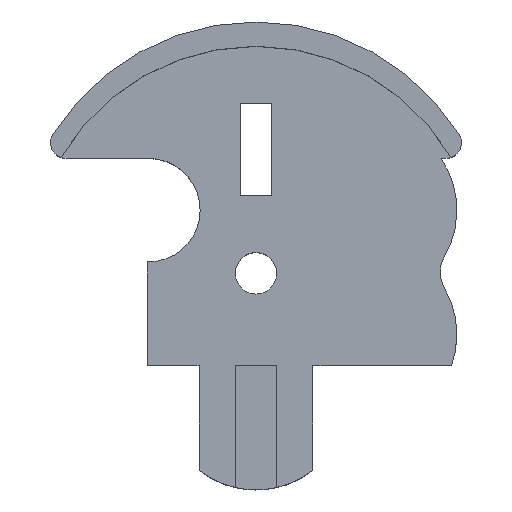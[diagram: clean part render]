
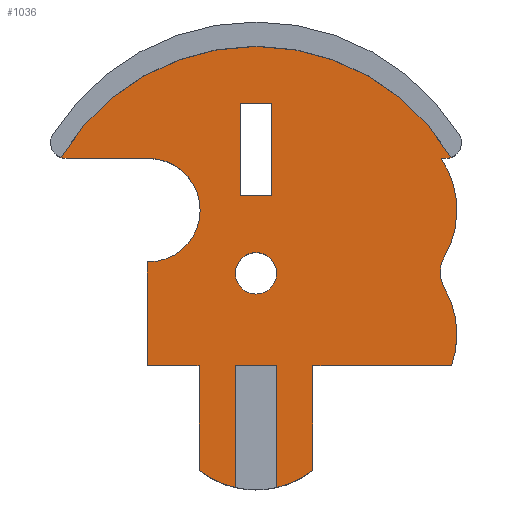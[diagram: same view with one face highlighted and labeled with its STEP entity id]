
A CAD part, top view. The second image highlights one B-rep face of the part: STEP entity #1036.
In plain terms, the highlighted planar face has unit normal (0, 0, 1).
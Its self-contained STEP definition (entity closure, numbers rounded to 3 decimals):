
#73=CARTESIAN_POINT('',(18.831,-0.817,10.0));
#74=VERTEX_POINT('',#73);
#75=CARTESIAN_POINT('',(-18.831,-0.817,10.0));
#76=VERTEX_POINT('',#75);
#77=CARTESIAN_POINT('',(0.0,-11.997,10.0));
#78=DIRECTION('',(0.0,0.0,1.0));
#79=DIRECTION('',(-0.86,-0.51,0.0));
#80=AXIS2_PLACEMENT_3D('',#77,#78,#79);
#81=CIRCLE('',#80,21.9);
#82=EDGE_CURVE('',#74,#76,#81,.T.);
#205=CARTESIAN_POINT('',(-1.998,-32.676,10.0));
#206=VERTEX_POINT('',#205);
#207=CARTESIAN_POINT('',(-1.998,-20.9,10.0));
#208=VERTEX_POINT('',#207);
#209=CARTESIAN_POINT('',(-1.998,-32.676,10.0));
#210=DIRECTION('',(0.0,1.0,0.0));
#211=VECTOR('',#210,11.775);
#212=LINE('',#209,#211);
#213=EDGE_CURVE('',#206,#208,#212,.T.);
#248=CARTESIAN_POINT('',(2.002,-20.9,10.0));
#249=VERTEX_POINT('',#248);
#250=CARTESIAN_POINT('',(2.002,-32.675,10.0));
#251=VERTEX_POINT('',#250);
#252=CARTESIAN_POINT('',(2.002,-20.9,10.0));
#253=DIRECTION('',(0.0,-1.0,0.0));
#254=VECTOR('',#253,11.774);
#255=LINE('',#252,#254);
#256=EDGE_CURVE('',#249,#251,#255,.T.);
#291=CARTESIAN_POINT('',(-1.998,-20.9,10.0));
#292=DIRECTION('',(1.0,0.0,0.0));
#293=VECTOR('',#292,4.0);
#294=LINE('',#291,#293);
#295=EDGE_CURVE('',#208,#249,#294,.T.);
#334=CARTESIAN_POINT('',(-5.5,-31.024,10.0));
#335=VERTEX_POINT('',#334);
#336=CARTESIAN_POINT('',(0.,-23.9,10.0));
#337=DIRECTION('',(0.0,0.0,1.0));
#338=DIRECTION('',(-0.611,-0.792,0.0));
#339=AXIS2_PLACEMENT_3D('',#336,#337,#338);
#340=CIRCLE('',#339,9.);
#341=EDGE_CURVE('',#335,#206,#340,.T.);
#360=CARTESIAN_POINT('',(5.5,-31.024,10.0));
#361=VERTEX_POINT('',#360);
#368=CARTESIAN_POINT('',(0.,-23.9,10.0));
#369=DIRECTION('',(0.0,0.0,1.0));
#370=DIRECTION('',(-0.611,-0.792,0.0));
#371=AXIS2_PLACEMENT_3D('',#368,#369,#370);
#372=CIRCLE('',#371,9.);
#373=EDGE_CURVE('',#251,#361,#372,.T.);
#393=CARTESIAN_POINT('',(1.5,4.426,10.0));
#394=VERTEX_POINT('',#393);
#401=CARTESIAN_POINT('',(-1.5,4.426,10.0));
#402=VERTEX_POINT('',#401);
#403=CARTESIAN_POINT('',(-1.5,4.426,10.0));
#404=DIRECTION('',(1.0,0.0,0.0));
#405=VECTOR('',#404,3.);
#406=LINE('',#403,#405);
#407=EDGE_CURVE('',#402,#394,#406,.T.);
#431=CARTESIAN_POINT('',(1.5,-4.532,10.0));
#432=VERTEX_POINT('',#431);
#439=CARTESIAN_POINT('',(1.5,4.426,10.0));
#440=DIRECTION('',(0.0,-1.0,0.0));
#441=VECTOR('',#440,8.958);
#442=LINE('',#439,#441);
#443=EDGE_CURVE('',#394,#432,#442,.T.);
#462=CARTESIAN_POINT('',(-1.5,-4.532,10.0));
#463=VERTEX_POINT('',#462);
#470=CARTESIAN_POINT('',(1.5,-4.532,10.0));
#471=DIRECTION('',(-1.0,0.0,0.0));
#472=VECTOR('',#471,3.);
#473=LINE('',#470,#472);
#474=EDGE_CURVE('',#432,#463,#473,.T.);
#492=CARTESIAN_POINT('',(-1.5,-4.532,10.0));
#493=DIRECTION('',(0.0,1.0,0.0));
#494=VECTOR('',#493,8.958);
#495=LINE('',#492,#494);
#496=EDGE_CURVE('',#463,#402,#495,.T.);
#507=CARTESIAN_POINT('',(2.0,-11.997,10.0));
#508=VERTEX_POINT('',#507);
#509=CARTESIAN_POINT('',(0.0,-11.997,10.0));
#510=DIRECTION('',(0.0,0.0,-1.0));
#511=DIRECTION('',(-1.0,0.0,0.0));
#512=AXIS2_PLACEMENT_3D('',#509,#510,#511);
#513=CIRCLE('',#512,2.0);
#514=EDGE_CURVE('',#508,#508,#513,.T.);
#545=CARTESIAN_POINT('',(18.878,-20.9,10.0));
#546=VERTEX_POINT('',#545);
#553=CARTESIAN_POINT('',(5.5,-20.9,10.0));
#554=VERTEX_POINT('',#553);
#555=CARTESIAN_POINT('',(5.5,-20.9,10.0));
#556=DIRECTION('',(1.0,0.0,0.0));
#557=VECTOR('',#556,13.378);
#558=LINE('',#555,#557);
#559=EDGE_CURVE('',#554,#546,#558,.T.);
#582=CARTESIAN_POINT('',(5.5,-31.024,10.0));
#583=DIRECTION('',(0.0,1.0,0.0));
#584=VECTOR('',#583,10.124);
#585=LINE('',#582,#584);
#586=EDGE_CURVE('',#361,#554,#585,.T.);
#609=CARTESIAN_POINT('',(-5.5,-20.9,10.0));
#610=VERTEX_POINT('',#609);
#611=CARTESIAN_POINT('',(-5.5,-20.9,10.0));
#612=DIRECTION('',(0.0,-1.0,0.0));
#613=VECTOR('',#612,10.124);
#614=LINE('',#611,#613);
#615=EDGE_CURVE('',#610,#335,#614,.T.);
#643=CARTESIAN_POINT('',(-10.5,-20.9,10.0));
#644=VERTEX_POINT('',#643);
#645=CARTESIAN_POINT('',(-10.5,-20.9,10.0));
#646=DIRECTION('',(1.0,0.0,0.0));
#647=VECTOR('',#646,5.);
#648=LINE('',#645,#647);
#649=EDGE_CURVE('',#644,#610,#648,.T.);
#674=CARTESIAN_POINT('',(-10.5,-10.9,10.0));
#675=VERTEX_POINT('',#674);
#676=CARTESIAN_POINT('',(-10.5,-10.9,10.0));
#677=DIRECTION('',(0.0,-1.0,0.0));
#678=VECTOR('',#677,10.);
#679=LINE('',#676,#678);
#680=EDGE_CURVE('',#675,#644,#679,.T.);
#705=CARTESIAN_POINT('',(-10.392,-10.9,10.0));
#706=VERTEX_POINT('',#705);
#707=CARTESIAN_POINT('',(-10.392,-10.9,10.0));
#708=DIRECTION('',(-1.0,0.0,0.0));
#709=VECTOR('',#708,0.108);
#710=LINE('',#707,#709);
#711=EDGE_CURVE('',#706,#675,#710,.T.);
#737=CARTESIAN_POINT('',(-10.392,-0.9,10.0));
#738=VERTEX_POINT('',#737);
#739=CARTESIAN_POINT('',(-10.392,-5.9,10.0));
#740=DIRECTION('',(0.0,0.0,-1.0));
#741=DIRECTION('',(0.0,1.0,0.0));
#742=AXIS2_PLACEMENT_3D('',#739,#740,#741);
#743=CIRCLE('',#742,5.);
#744=EDGE_CURVE('',#738,#706,#743,.T.);
#769=CARTESIAN_POINT('',(-18.34,-0.9,10.0));
#770=VERTEX_POINT('',#769);
#771=CARTESIAN_POINT('',(-18.34,-0.9,10.0));
#772=DIRECTION('',(1.0,0.0,0.0));
#773=VECTOR('',#772,7.948);
#774=LINE('',#771,#773);
#775=EDGE_CURVE('',#770,#738,#774,.T.);
#801=CARTESIAN_POINT('',(-18.34,0.6,10.0));
#802=DIRECTION('',(0.0,0.0,1.0));
#803=DIRECTION('',(-0.847,0.531,0.0));
#804=AXIS2_PLACEMENT_3D('',#801,#802,#803);
#805=CIRCLE('',#804,1.5);
#806=EDGE_CURVE('',#76,#770,#805,.T.);
#861=CARTESIAN_POINT('',(18.34,-0.9,10.0));
#862=VERTEX_POINT('',#861);
#863=CARTESIAN_POINT('',(18.34,0.6,10.0));
#864=DIRECTION('',(0.0,0.0,1.0));
#865=DIRECTION('',(0.0,-1.0,0.0));
#866=AXIS2_PLACEMENT_3D('',#863,#864,#865);
#867=CIRCLE('',#866,1.5);
#868=EDGE_CURVE('',#862,#74,#867,.T.);
#893=CARTESIAN_POINT('',(17.876,-0.9,10.0));
#894=VERTEX_POINT('',#893);
#895=CARTESIAN_POINT('',(17.876,-0.9,10.0));
#896=DIRECTION('',(1.0,0.0,0.0));
#897=VECTOR('',#896,0.464);
#898=LINE('',#895,#897);
#899=EDGE_CURVE('',#894,#862,#898,.T.);
#925=CARTESIAN_POINT('',(18.187,-10.4,10.0));
#926=VERTEX_POINT('',#925);
#927=CARTESIAN_POINT('',(10.392,-5.9,10.0));
#928=DIRECTION('',(0.0,0.0,1.0));
#929=DIRECTION('',(0.866,-0.5,0.0));
#930=AXIS2_PLACEMENT_3D('',#927,#928,#929);
#931=CIRCLE('',#930,9.0);
#932=EDGE_CURVE('',#926,#894,#931,.T.);
#958=CARTESIAN_POINT('',(18.187,-13.4,10.0));
#959=VERTEX_POINT('',#958);
#960=CARTESIAN_POINT('',(20.785,-11.9,10.0));
#961=DIRECTION('',(0.0,0.0,-1.0));
#962=DIRECTION('',(0.866,-0.5,0.0));
#963=AXIS2_PLACEMENT_3D('',#960,#961,#962);
#964=CIRCLE('',#963,3.);
#965=EDGE_CURVE('',#959,#926,#964,.T.);
#989=CARTESIAN_POINT('',(10.392,-17.9,10.0));
#990=DIRECTION('',(0.0,0.0,1.0));
#991=DIRECTION('',(0.943,-0.333,0.0));
#992=AXIS2_PLACEMENT_3D('',#989,#990,#991);
#993=CIRCLE('',#992,9.0);
#994=EDGE_CURVE('',#546,#959,#993,.T.);
#1000=CARTESIAN_POINT('',(0.913,-9.783,10.0));
#1001=DIRECTION('',(0.0,0.0,1.0));
#1002=DIRECTION('',(1.0,0.0,0.0));
#1003=AXIS2_PLACEMENT_3D('',#1000,#1001,#1002);
#1004=PLANE('',#1003);
#1005=ORIENTED_EDGE('',*,*,#82,.T.);
#1006=ORIENTED_EDGE('',*,*,#806,.T.);
#1007=ORIENTED_EDGE('',*,*,#775,.T.);
#1008=ORIENTED_EDGE('',*,*,#744,.T.);
#1009=ORIENTED_EDGE('',*,*,#711,.T.);
#1010=ORIENTED_EDGE('',*,*,#680,.T.);
#1011=ORIENTED_EDGE('',*,*,#649,.T.);
#1012=ORIENTED_EDGE('',*,*,#615,.T.);
#1013=ORIENTED_EDGE('',*,*,#341,.T.);
#1014=ORIENTED_EDGE('',*,*,#213,.T.);
#1015=ORIENTED_EDGE('',*,*,#295,.T.);
#1016=ORIENTED_EDGE('',*,*,#256,.T.);
#1017=ORIENTED_EDGE('',*,*,#373,.T.);
#1018=ORIENTED_EDGE('',*,*,#586,.T.);
#1019=ORIENTED_EDGE('',*,*,#559,.T.);
#1020=ORIENTED_EDGE('',*,*,#994,.T.);
#1021=ORIENTED_EDGE('',*,*,#965,.T.);
#1022=ORIENTED_EDGE('',*,*,#932,.T.);
#1023=ORIENTED_EDGE('',*,*,#899,.T.);
#1024=ORIENTED_EDGE('',*,*,#868,.T.);
#1025=EDGE_LOOP('',(#1005,#1006,#1007,#1008,#1009,#1010,#1011,#1012,#1013,#1014,#1015,#1016,#1017,#1018,#1019,#1020,#1021,#1022,#1023,#1024));
#1026=FACE_OUTER_BOUND('',#1025,.T.);
#1027=ORIENTED_EDGE('',*,*,#407,.T.);
#1028=ORIENTED_EDGE('',*,*,#443,.T.);
#1029=ORIENTED_EDGE('',*,*,#474,.T.);
#1030=ORIENTED_EDGE('',*,*,#496,.T.);
#1031=EDGE_LOOP('',(#1027,#1028,#1029,#1030));
#1032=FACE_BOUND('',#1031,.T.);
#1033=ORIENTED_EDGE('',*,*,#514,.T.);
#1034=EDGE_LOOP('',(#1033));
#1035=FACE_BOUND('',#1034,.T.);
#1036=ADVANCED_FACE('',(#1026,#1032,#1035),#1004,.T.);
